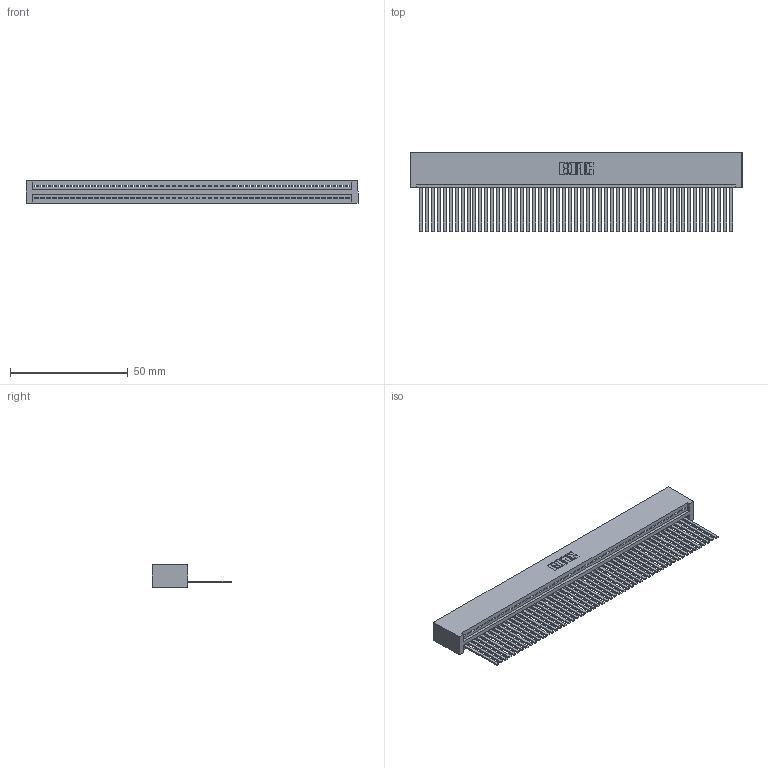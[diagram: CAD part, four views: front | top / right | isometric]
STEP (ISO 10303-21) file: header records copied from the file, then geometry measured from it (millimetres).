
FILE_DESCRIPTION (( 'STEP AP203' ), '1' );
FILE_NAME ('345-053-544-101.STEP', '2018-09-23T18:43:53', ( '' ), ( '' ), 'SwSTEP 2.0', 'SolidWorks 2016', '' );
FILE_SCHEMA (( 'CONFIG_CONTROL_DESIGN' ));
Length unit declared in the file: inch
Products named in the file (3): 345-053-544-101; 345 Part_No Mounting Lugs; 345-292-001_345-293-144
Assembly tree (54 placements, depth 2):
  345-053-544-101
    345 Part_No Mounting Lugs
    345-292-001_345-293-144  x53
Bounding box: 141.22 x 33.96 x 9.4 mm (x, y, z)
Volume: 14701.9 mm3; surface area: 21719.8 mm2
Topology: 54 solids, 54 shells, 2874 faces, 8691 edges, 5722 vertices
Faces by surface type: plane 1984, cylinder 890
Entity records: 37947 total; most frequent: CARTESIAN_POINT 6579, ORIENTED_EDGE 6566, DIRECTION 5721, EDGE_CURVE 3283, VECTOR 2951, LINE 2951, VERTEX_POINT 2186, AXIS2_PLACEMENT_3D 1385
